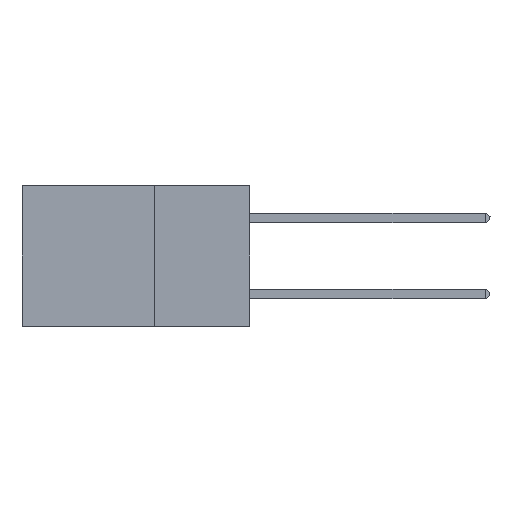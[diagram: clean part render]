
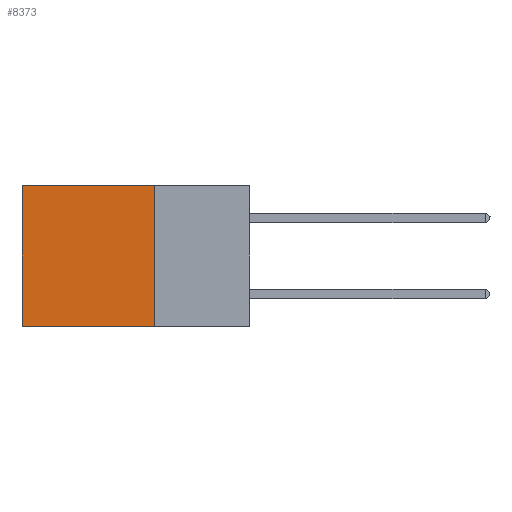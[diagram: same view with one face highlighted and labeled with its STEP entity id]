
A CAD part, left-side view. The second image highlights one B-rep face of the part: STEP entity #8373.
In plain terms, the highlighted planar face has unit normal (-1, 0, 0).
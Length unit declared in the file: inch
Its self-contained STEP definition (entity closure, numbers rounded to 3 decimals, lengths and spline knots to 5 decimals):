
#211 = CARTESIAN_POINT ( 'NONE',  ( 0.2875, 0.6, 0. ) ) ;
#317 = LINE ( 'NONE', #13735, #13353 ) ;
#1292 = VECTOR ( 'NONE', #9418, 39.37008 ) ;
#1918 = EDGE_LOOP ( 'NONE', ( #9466, #1989, #14095, #12817 ) ) ;
#1985 = DIRECTION ( 'NONE',  ( 1., 0., 0. ) ) ;
#1989 = ORIENTED_EDGE ( 'NONE', *, *, #9003, .F. ) ;
#2165 = LINE ( 'NONE', #6974, #10391 ) ;
#3647 = LINE ( 'NONE', #13464, #15045 ) ;
#4934 = DIRECTION ( 'NONE',  ( 0., 1., 0. ) ) ;
#5832 = PLANE ( 'NONE',  #8986 ) ;
#6959 = VERTEX_POINT ( 'NONE', #9333 ) ;
#6974 = CARTESIAN_POINT ( 'NONE',  ( 0.2875, 0.6, 0. ) ) ;
#7024 = CARTESIAN_POINT ( 'NONE',  ( 0.2875, 0.25, -0.37 ) ) ;
#8373 = ADVANCED_FACE ( 'NONE', ( #13076 ), #5832, .F. ) ;
#8678 = CARTESIAN_POINT ( 'NONE',  ( 0.2875, 0.6, -0.37 ) ) ;
#8785 = EDGE_CURVE ( 'NONE', #6959, #13007, #10321, .T. ) ;
#8986 = AXIS2_PLACEMENT_3D ( 'NONE', #9439, #1985, #15561 ) ;
#9003 = EDGE_CURVE ( 'NONE', #11335, #14798, #3647, .T. ) ;
#9333 = CARTESIAN_POINT ( 'NONE',  ( 0.2875, 0.25, 0. ) ) ;
#9418 = DIRECTION ( 'NONE',  ( 0., 1., 0. ) ) ;
#9439 = CARTESIAN_POINT ( 'NONE',  ( 0.2875, 0.25, 0. ) ) ;
#9466 = ORIENTED_EDGE ( 'NONE', *, *, #12351, .T. ) ;
#10321 = LINE ( 'NONE', #15222, #1292 ) ;
#10336 = DIRECTION ( 'NONE',  ( 0., 0., -1. ) ) ;
#10391 = VECTOR ( 'NONE', #10672, 39.37008 ) ;
#10672 = DIRECTION ( 'NONE',  ( 0., 0., -1. ) ) ;
#11335 = VERTEX_POINT ( 'NONE', #7024 ) ;
#12351 = EDGE_CURVE ( 'NONE', #13007, #14798, #2165, .T. ) ;
#12817 = ORIENTED_EDGE ( 'NONE', *, *, #8785, .T. ) ;
#13007 = VERTEX_POINT ( 'NONE', #211 ) ;
#13076 = FACE_OUTER_BOUND ( 'NONE', #1918, .T. ) ;
#13353 = VECTOR ( 'NONE', #10336, 39.37008 ) ;
#13464 = CARTESIAN_POINT ( 'NONE',  ( 0.2875, 0.25, -0.37 ) ) ;
#13735 = CARTESIAN_POINT ( 'NONE',  ( 0.2875, 0.25, 0. ) ) ;
#13914 = EDGE_CURVE ( 'NONE', #6959, #11335, #317, .T. ) ;
#14095 = ORIENTED_EDGE ( 'NONE', *, *, #13914, .F. ) ;
#14798 = VERTEX_POINT ( 'NONE', #8678 ) ;
#15045 = VECTOR ( 'NONE', #4934, 39.37008 ) ;
#15222 = CARTESIAN_POINT ( 'NONE',  ( 0.2875, 0.25, 0. ) ) ;
#15561 = DIRECTION ( 'NONE',  ( 0., 0., -1. ) ) ;
